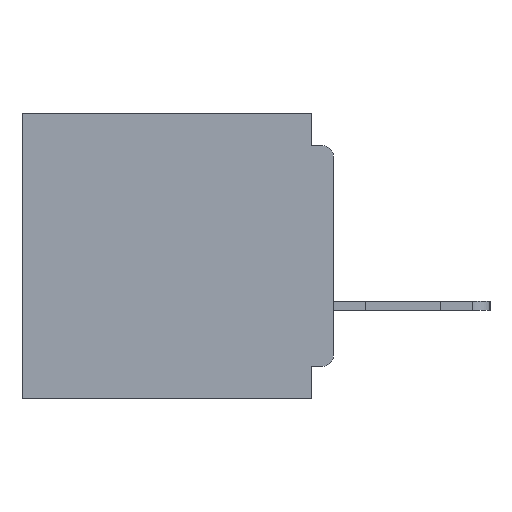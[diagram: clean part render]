
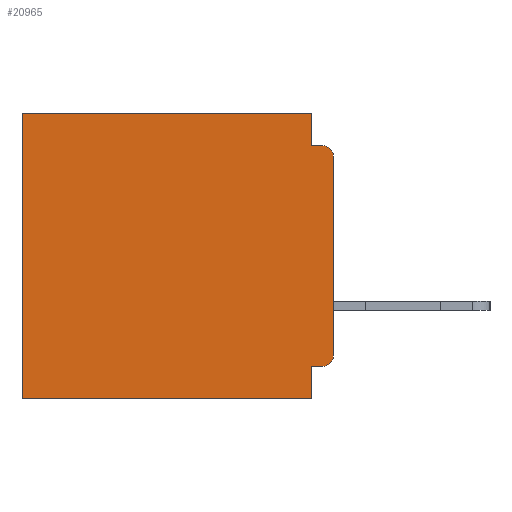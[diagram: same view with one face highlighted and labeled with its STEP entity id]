
A CAD part, left-side view. The second image highlights one B-rep face of the part: STEP entity #20965.
In plain terms, the highlighted planar face has unit normal (-1, 0, 0).
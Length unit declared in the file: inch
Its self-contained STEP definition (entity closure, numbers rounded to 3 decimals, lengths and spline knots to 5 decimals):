
#48 = ORIENTED_EDGE ( 'NONE', *, *, #7517, .F. ) ;
#102 = DIRECTION ( 'NONE',  ( 0., 1., 0. ) ) ;
#2244 = ORIENTED_EDGE ( 'NONE', *, *, #19261, .F. ) ;
#2312 = LINE ( 'NONE', #44204, #20972 ) ;
#2937 = PLANE ( 'NONE',  #18765 ) ;
#3019 = LINE ( 'NONE', #27331, #43974 ) ;
#3593 = DIRECTION ( 'NONE',  ( 0., 0., -1. ) ) ;
#4362 = VERTEX_POINT ( 'NONE', #27005 ) ;
#4491 = VERTEX_POINT ( 'NONE', #17790 ) ;
#4861 = DIRECTION ( 'NONE',  ( 0., -1., 0. ) ) ;
#5989 = LINE ( 'NONE', #8007, #25820 ) ;
#6262 = CARTESIAN_POINT ( 'NONE',  ( 0.3, 0., -0.4 ) ) ;
#6572 = AXIS2_PLACEMENT_3D ( 'NONE', #33799, #10102, #37822 ) ;
#6783 = VERTEX_POINT ( 'NONE', #42873 ) ;
#6981 = DIRECTION ( 'NONE',  ( 1., 0., 0. ) ) ;
#7517 = EDGE_CURVE ( 'NONE', #50495, #13825, #40916, .T. ) ;
#7795 = DIRECTION ( 'NONE',  ( 0., 0., -1. ) ) ;
#8007 = CARTESIAN_POINT ( 'NONE',  ( 0.3, 0., 0. ) ) ;
#10102 = DIRECTION ( 'NONE',  ( -1., 0., 0. ) ) ;
#10482 = ORIENTED_EDGE ( 'NONE', *, *, #22918, .T. ) ;
#11341 = CARTESIAN_POINT ( 'NONE',  ( 0.3, 0.437, -0.4 ) ) ;
#12619 = CARTESIAN_POINT ( 'NONE',  ( 0.3, 0.031, -0.355 ) ) ;
#12852 = EDGE_CURVE ( 'NONE', #15916, #28552, #3019, .T. ) ;
#13825 = VERTEX_POINT ( 'NONE', #18333 ) ;
#14280 = CARTESIAN_POINT ( 'NONE',  ( 0.3, 0.015, -0.045 ) ) ;
#15916 = VERTEX_POINT ( 'NONE', #37498 ) ;
#15958 = VECTOR ( 'NONE', #32904, 39.37008 ) ;
#16154 = VERTEX_POINT ( 'NONE', #11341 ) ;
#16217 = DIRECTION ( 'NONE',  ( 0., 1., 0. ) ) ;
#16255 = VECTOR ( 'NONE', #16217, 39.37008 ) ;
#17790 = CARTESIAN_POINT ( 'NONE',  ( 0.3, 0., -0.34 ) ) ;
#18055 = DIRECTION ( 'NONE',  ( 0., 0., -1. ) ) ;
#18333 = CARTESIAN_POINT ( 'NONE',  ( 0.3, 0.031, -0.4 ) ) ;
#18620 = VECTOR ( 'NONE', #7795, 39.37008 ) ;
#18765 = AXIS2_PLACEMENT_3D ( 'NONE', #42340, #6981, #34699 ) ;
#19261 = EDGE_CURVE ( 'NONE', #28552, #49607, #2312, .T. ) ;
#20555 = ORIENTED_EDGE ( 'NONE', *, *, #45737, .F. ) ;
#20965 = ADVANCED_FACE ( 'NONE', ( #35718 ), #2937, .F. ) ;
#20972 = VECTOR ( 'NONE', #4861, 39.37008 ) ;
#22918 = EDGE_CURVE ( 'NONE', #6783, #4491, #36132, .T. ) ;
#23531 = VERTEX_POINT ( 'NONE', #39302 ) ;
#23614 = DIRECTION ( 'NONE',  ( -1., 0., 0. ) ) ;
#23635 = ORIENTED_EDGE ( 'NONE', *, *, #44684, .F. ) ;
#24652 = EDGE_LOOP ( 'NONE', ( #20555, #49955, #2244, #44258, #36433, #25103, #23635, #48, #28383, #10482 ) ) ;
#25103 = ORIENTED_EDGE ( 'NONE', *, *, #46308, .T. ) ;
#25467 = LINE ( 'NONE', #32082, #16255 ) ;
#25820 = VECTOR ( 'NONE', #102, 39.37008 ) ;
#26338 = DIRECTION ( 'NONE',  ( 0., 0., -1. ) ) ;
#27005 = CARTESIAN_POINT ( 'NONE',  ( 0.3, 0.437, 0. ) ) ;
#27331 = CARTESIAN_POINT ( 'NONE',  ( 0.3, 0.031, 0. ) ) ;
#28144 = VECTOR ( 'NONE', #18055, 39.37008 ) ;
#28383 = ORIENTED_EDGE ( 'NONE', *, *, #49259, .F. ) ;
#28552 = VERTEX_POINT ( 'NONE', #46697 ) ;
#28912 = CARTESIAN_POINT ( 'NONE',  ( 0.3, 0., -0.4 ) ) ;
#32082 = CARTESIAN_POINT ( 'NONE',  ( 0.3, 0., -0.355 ) ) ;
#32904 = DIRECTION ( 'NONE',  ( 0., 1., 0. ) ) ;
#33799 = CARTESIAN_POINT ( 'NONE',  ( 0.3, 0.015, -0.06 ) ) ;
#34699 = DIRECTION ( 'NONE',  ( 0., 0., -1. ) ) ;
#35703 = LINE ( 'NONE', #6262, #46196 ) ;
#35718 = FACE_OUTER_BOUND ( 'NONE', #24652, .T. ) ;
#36132 = CIRCLE ( 'NONE', #47243, 0.015 ) ;
#36144 = EDGE_CURVE ( 'NONE', #23531, #49607, #44227, .T. ) ;
#36433 = ORIENTED_EDGE ( 'NONE', *, *, #44514, .T. ) ;
#37498 = CARTESIAN_POINT ( 'NONE',  ( 0.3, 0.031, 0. ) ) ;
#37769 = CARTESIAN_POINT ( 'NONE',  ( 0.3, 0.437, -0.4 ) ) ;
#37822 = DIRECTION ( 'NONE',  ( 0., 0., -1. ) ) ;
#38248 = LINE ( 'NONE', #28912, #15958 ) ;
#38759 = LINE ( 'NONE', #37769, #28144 ) ;
#39302 = CARTESIAN_POINT ( 'NONE',  ( 0.3, 0., -0.06 ) ) ;
#39354 = CARTESIAN_POINT ( 'NONE',  ( 0.3, 0.031, -0.4 ) ) ;
#40916 = LINE ( 'NONE', #39354, #18620 ) ;
#42340 = CARTESIAN_POINT ( 'NONE',  ( 0.3, 0., -0.4 ) ) ;
#42873 = CARTESIAN_POINT ( 'NONE',  ( 0.3, 0.015, -0.355 ) ) ;
#43974 = VECTOR ( 'NONE', #3593, 39.37008 ) ;
#44204 = CARTESIAN_POINT ( 'NONE',  ( 0.3, 0., -0.045 ) ) ;
#44227 = CIRCLE ( 'NONE', #6572, 0.015 ) ;
#44258 = ORIENTED_EDGE ( 'NONE', *, *, #12852, .F. ) ;
#44514 = EDGE_CURVE ( 'NONE', #15916, #4362, #5989, .T. ) ;
#44684 = EDGE_CURVE ( 'NONE', #13825, #16154, #38248, .T. ) ;
#45737 = EDGE_CURVE ( 'NONE', #23531, #4491, #35703, .T. ) ;
#46196 = VECTOR ( 'NONE', #26338, 39.37008 ) ;
#46308 = EDGE_CURVE ( 'NONE', #4362, #16154, #38759, .T. ) ;
#46697 = CARTESIAN_POINT ( 'NONE',  ( 0.3, 0.031, -0.045 ) ) ;
#47230 = CARTESIAN_POINT ( 'NONE',  ( 0.3, 0.015, -0.34 ) ) ;
#47243 = AXIS2_PLACEMENT_3D ( 'NONE', #47230, #23614, #51108 ) ;
#49259 = EDGE_CURVE ( 'NONE', #6783, #50495, #25467, .T. ) ;
#49607 = VERTEX_POINT ( 'NONE', #14280 ) ;
#49955 = ORIENTED_EDGE ( 'NONE', *, *, #36144, .T. ) ;
#50495 = VERTEX_POINT ( 'NONE', #12619 ) ;
#51108 = DIRECTION ( 'NONE',  ( 0., 0., -1. ) ) ;
